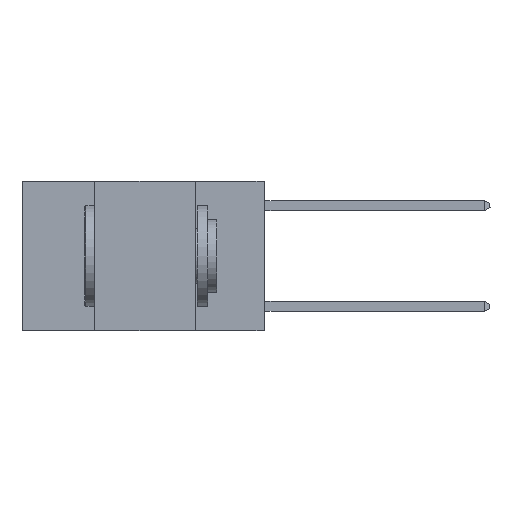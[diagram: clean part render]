
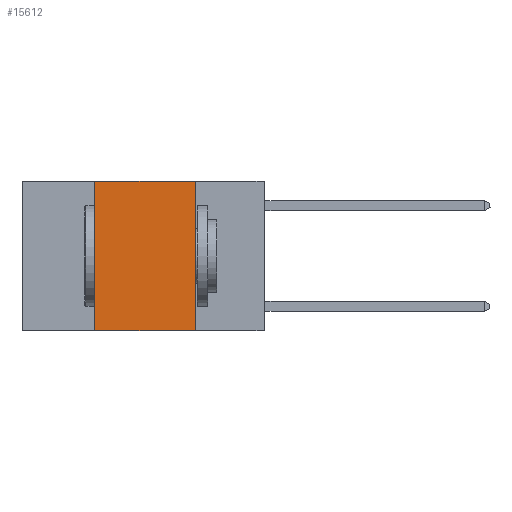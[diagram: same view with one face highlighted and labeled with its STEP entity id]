
A CAD part, left-side view. The second image highlights one B-rep face of the part: STEP entity #15612.
In plain terms, the highlighted planar face has unit normal (-1, 0, 0).
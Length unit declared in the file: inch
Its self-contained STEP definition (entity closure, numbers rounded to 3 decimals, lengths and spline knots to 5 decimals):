
#1372 = DIRECTION ( 'NONE',  ( 1., 0., 0. ) ) ;
#2092 = EDGE_CURVE ( 'NONE', #5421, #13997, #27854, .T. ) ;
#2939 = CARTESIAN_POINT ( 'NONE',  ( 0., 0.42, -0.37 ) ) ;
#4517 = ORIENTED_EDGE ( 'NONE', *, *, #27262, .F. ) ;
#5232 = DIRECTION ( 'NONE',  ( 0., -1., 0. ) ) ;
#5421 = VERTEX_POINT ( 'NONE', #16783 ) ;
#5513 = CARTESIAN_POINT ( 'NONE',  ( 0., 0.42, 0. ) ) ;
#6013 = ORIENTED_EDGE ( 'NONE', *, *, #2092, .F. ) ;
#7335 = AXIS2_PLACEMENT_3D ( 'NONE', #20312, #1372, #17995 ) ;
#8797 = VECTOR ( 'NONE', #16959, 39.37008 ) ;
#10590 = VECTOR ( 'NONE', #19244, 39.37008 ) ;
#10802 = PLANE ( 'NONE',  #7335 ) ;
#12318 = LINE ( 'NONE', #5513, #24266 ) ;
#13997 = VERTEX_POINT ( 'NONE', #19637 ) ;
#14055 = VECTOR ( 'NONE', #5232, 39.37008 ) ;
#14739 = VERTEX_POINT ( 'NONE', #2939 ) ;
#15147 = ORIENTED_EDGE ( 'NONE', *, *, #19615, .T. ) ;
#15612 = ADVANCED_FACE ( 'NONE', ( #21964 ), #10802, .F. ) ;
#16288 = VERTEX_POINT ( 'NONE', #29634 ) ;
#16474 = CARTESIAN_POINT ( 'NONE',  ( 0., 0.17, 0. ) ) ;
#16783 = CARTESIAN_POINT ( 'NONE',  ( 0., 0.17, 0. ) ) ;
#16810 = CARTESIAN_POINT ( 'NONE',  ( 0., 0.6, -0.37 ) ) ;
#16959 = DIRECTION ( 'NONE',  ( 0., 0., -1. ) ) ;
#17090 = CARTESIAN_POINT ( 'NONE',  ( 0., 0.6, 0. ) ) ;
#17995 = DIRECTION ( 'NONE',  ( 0., 0., -1. ) ) ;
#19244 = DIRECTION ( 'NONE',  ( 0., -1., 0. ) ) ;
#19475 = EDGE_LOOP ( 'NONE', ( #6013, #22256, #4517, #15147 ) ) ;
#19615 = EDGE_CURVE ( 'NONE', #14739, #13997, #22511, .T. ) ;
#19637 = CARTESIAN_POINT ( 'NONE',  ( 0., 0.17, -0.37 ) ) ;
#20312 = CARTESIAN_POINT ( 'NONE',  ( 0., 0.6, 0. ) ) ;
#20418 = LINE ( 'NONE', #17090, #14055 ) ;
#21964 = FACE_OUTER_BOUND ( 'NONE', #19475, .T. ) ;
#22149 = DIRECTION ( 'NONE',  ( 0., 0., 1. ) ) ;
#22256 = ORIENTED_EDGE ( 'NONE', *, *, #23851, .F. ) ;
#22511 = LINE ( 'NONE', #16810, #10590 ) ;
#23851 = EDGE_CURVE ( 'NONE', #16288, #5421, #20418, .T. ) ;
#24266 = VECTOR ( 'NONE', #22149, 39.37008 ) ;
#27262 = EDGE_CURVE ( 'NONE', #14739, #16288, #12318, .T. ) ;
#27854 = LINE ( 'NONE', #16474, #8797 ) ;
#29634 = CARTESIAN_POINT ( 'NONE',  ( 0., 0.42, 0. ) ) ;
